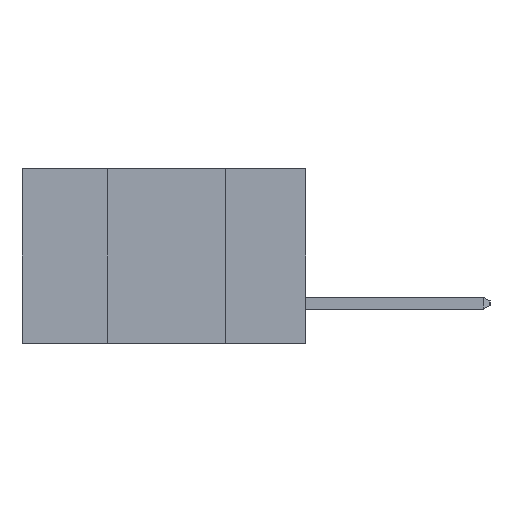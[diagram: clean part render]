
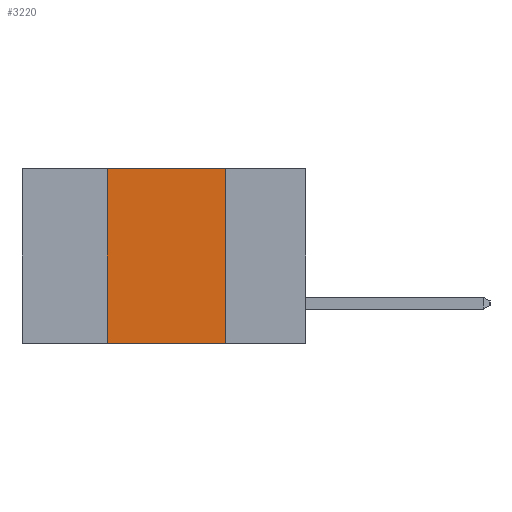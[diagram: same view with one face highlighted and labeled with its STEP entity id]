
A CAD part, left-side view. The second image highlights one B-rep face of the part: STEP entity #3220.
In plain terms, the highlighted planar face has unit normal (-1, 0, 0).
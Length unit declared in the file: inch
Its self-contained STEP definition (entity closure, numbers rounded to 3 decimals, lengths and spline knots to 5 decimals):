
#1673 = FACE_OUTER_BOUND ( 'NONE', #11341, .T. ) ;
#1905 = VECTOR ( 'NONE', #10493, 39.37008 ) ;
#2816 = VERTEX_POINT ( 'NONE', #7147 ) ;
#3034 = DIRECTION ( 'NONE',  ( 0., -1., 0. ) ) ;
#3062 = ORIENTED_EDGE ( 'NONE', *, *, #14384, .F. ) ;
#3220 = ADVANCED_FACE ( 'NONE', ( #1673 ), #10686, .F. ) ;
#3980 = ORIENTED_EDGE ( 'NONE', *, *, #14567, .F. ) ;
#4170 = LINE ( 'NONE', #10070, #13937 ) ;
#4215 = CARTESIAN_POINT ( 'NONE',  ( 0., 0.42, -0.37 ) ) ;
#4831 = CARTESIAN_POINT ( 'NONE',  ( 0., 0.17, -0.37 ) ) ;
#5071 = CARTESIAN_POINT ( 'NONE',  ( 0., 0.6, 0. ) ) ;
#5379 = DIRECTION ( 'NONE',  ( 0., 0., 1. ) ) ;
#6597 = VECTOR ( 'NONE', #13330, 39.37008 ) ;
#6802 = AXIS2_PLACEMENT_3D ( 'NONE', #12766, #9611, #9398 ) ;
#7147 = CARTESIAN_POINT ( 'NONE',  ( 0., 0.42, -0.37 ) ) ;
#7304 = VERTEX_POINT ( 'NONE', #11352 ) ;
#9317 = CARTESIAN_POINT ( 'NONE',  ( 0., 0.17, -0.37 ) ) ;
#9398 = DIRECTION ( 'NONE',  ( 0., 0., -1. ) ) ;
#9499 = VERTEX_POINT ( 'NONE', #4831 ) ;
#9611 = DIRECTION ( 'NONE',  ( 1., 0., 0. ) ) ;
#10070 = CARTESIAN_POINT ( 'NONE',  ( 0., 0.6, -0.37 ) ) ;
#10299 = EDGE_CURVE ( 'NONE', #2816, #9499, #4170, .T. ) ;
#10493 = DIRECTION ( 'NONE',  ( 0., 0., -1. ) ) ;
#10686 = PLANE ( 'NONE',  #6802 ) ;
#11246 = EDGE_CURVE ( 'NONE', #7304, #9499, #11340, .T. ) ;
#11340 = LINE ( 'NONE', #9317, #1905 ) ;
#11341 = EDGE_LOOP ( 'NONE', ( #11934, #3062, #3980, #13215 ) ) ;
#11352 = CARTESIAN_POINT ( 'NONE',  ( 0., 0.17, 0. ) ) ;
#11934 = ORIENTED_EDGE ( 'NONE', *, *, #11246, .F. ) ;
#12409 = VERTEX_POINT ( 'NONE', #12497 ) ;
#12478 = LINE ( 'NONE', #5071, #6597 ) ;
#12497 = CARTESIAN_POINT ( 'NONE',  ( 0., 0.42, 0. ) ) ;
#12766 = CARTESIAN_POINT ( 'NONE',  ( 0., 0.6, 0. ) ) ;
#13020 = LINE ( 'NONE', #4215, #13403 ) ;
#13215 = ORIENTED_EDGE ( 'NONE', *, *, #10299, .T. ) ;
#13330 = DIRECTION ( 'NONE',  ( 0., -1., 0. ) ) ;
#13403 = VECTOR ( 'NONE', #5379, 39.37008 ) ;
#13937 = VECTOR ( 'NONE', #3034, 39.37008 ) ;
#14384 = EDGE_CURVE ( 'NONE', #12409, #7304, #12478, .T. ) ;
#14567 = EDGE_CURVE ( 'NONE', #2816, #12409, #13020, .T. ) ;
